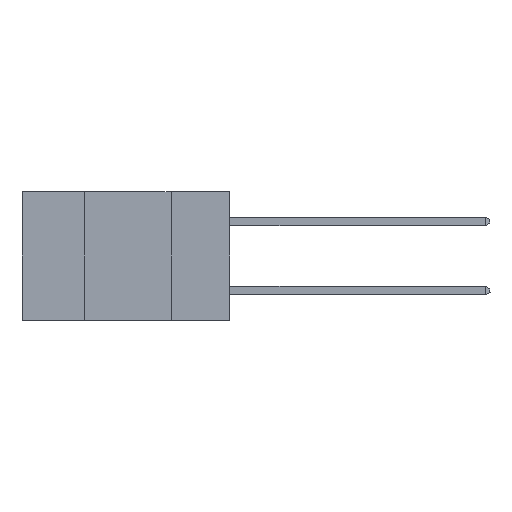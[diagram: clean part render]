
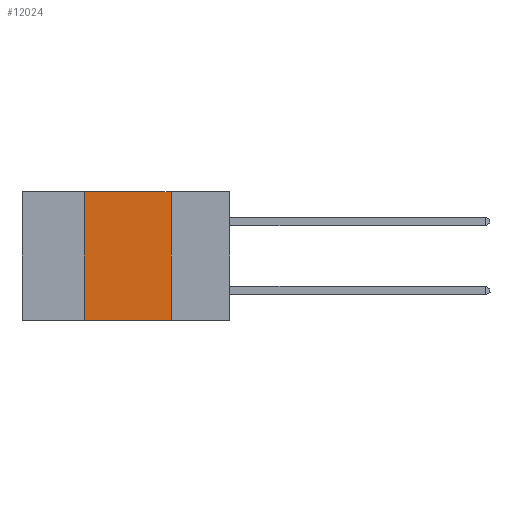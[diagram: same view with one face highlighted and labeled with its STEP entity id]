
A CAD part, left-side view. The second image highlights one B-rep face of the part: STEP entity #12024.
In plain terms, the highlighted planar face has unit normal (-1, 0, 0).
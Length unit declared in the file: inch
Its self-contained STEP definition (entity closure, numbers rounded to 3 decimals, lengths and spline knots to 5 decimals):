
#28 = CARTESIAN_POINT ( 'NONE',  ( 0., 0.42, 0. ) ) ;
#315 = CARTESIAN_POINT ( 'NONE',  ( 0., 0.17, -0.37 ) ) ;
#493 = PLANE ( 'NONE',  #7397 ) ;
#1319 = CARTESIAN_POINT ( 'NONE',  ( 0., 0.6, 0. ) ) ;
#1642 = CARTESIAN_POINT ( 'NONE',  ( 0., 0.6, 0. ) ) ;
#1688 = FACE_OUTER_BOUND ( 'NONE', #5638, .T. ) ;
#1733 = VERTEX_POINT ( 'NONE', #3827 ) ;
#1845 = CARTESIAN_POINT ( 'NONE',  ( 0., 0.17, 0. ) ) ;
#2666 = EDGE_CURVE ( 'NONE', #1733, #10525, #6916, .T. ) ;
#2946 = LINE ( 'NONE', #5832, #10233 ) ;
#3437 = ORIENTED_EDGE ( 'NONE', *, *, #8078, .F. ) ;
#3593 = ORIENTED_EDGE ( 'NONE', *, *, #2666, .F. ) ;
#3827 = CARTESIAN_POINT ( 'NONE',  ( 0., 0.42, -0.37 ) ) ;
#3886 = DIRECTION ( 'NONE',  ( 0., 0., -1. ) ) ;
#5344 = VECTOR ( 'NONE', #9890, 39.37008 ) ;
#5638 = EDGE_LOOP ( 'NONE', ( #3437, #11564, #3593, #10480 ) ) ;
#5804 = VECTOR ( 'NONE', #7996, 39.37008 ) ;
#5832 = CARTESIAN_POINT ( 'NONE',  ( 0., 0.6, -0.37 ) ) ;
#6435 = CARTESIAN_POINT ( 'NONE',  ( 0., 0.42, 0. ) ) ;
#6535 = VERTEX_POINT ( 'NONE', #12092 ) ;
#6916 = LINE ( 'NONE', #28, #5344 ) ;
#7397 = AXIS2_PLACEMENT_3D ( 'NONE', #1642, #9366, #3886 ) ;
#7996 = DIRECTION ( 'NONE',  ( 0., -1., 0. ) ) ;
#8078 = EDGE_CURVE ( 'NONE', #6535, #13246, #11946, .T. ) ;
#8098 = DIRECTION ( 'NONE',  ( 0., -1., 0. ) ) ;
#8146 = EDGE_CURVE ( 'NONE', #1733, #13246, #2946, .T. ) ;
#8459 = DIRECTION ( 'NONE',  ( 0., 0., -1. ) ) ;
#9366 = DIRECTION ( 'NONE',  ( 1., 0., 0. ) ) ;
#9890 = DIRECTION ( 'NONE',  ( 0., 0., 1. ) ) ;
#10233 = VECTOR ( 'NONE', #8098, 39.37008 ) ;
#10480 = ORIENTED_EDGE ( 'NONE', *, *, #8146, .T. ) ;
#10525 = VERTEX_POINT ( 'NONE', #6435 ) ;
#11564 = ORIENTED_EDGE ( 'NONE', *, *, #12559, .F. ) ;
#11618 = VECTOR ( 'NONE', #8459, 39.37008 ) ;
#11946 = LINE ( 'NONE', #1845, #11618 ) ;
#12024 = ADVANCED_FACE ( 'NONE', ( #1688 ), #493, .F. ) ;
#12092 = CARTESIAN_POINT ( 'NONE',  ( 0., 0.17, 0. ) ) ;
#12559 = EDGE_CURVE ( 'NONE', #10525, #6535, #12892, .T. ) ;
#12892 = LINE ( 'NONE', #1319, #5804 ) ;
#13246 = VERTEX_POINT ( 'NONE', #315 ) ;
